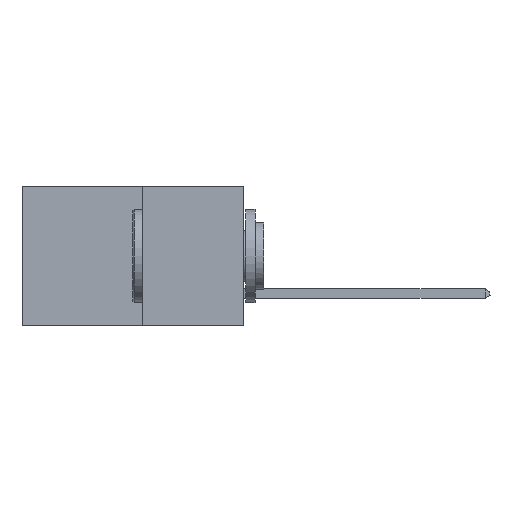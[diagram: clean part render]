
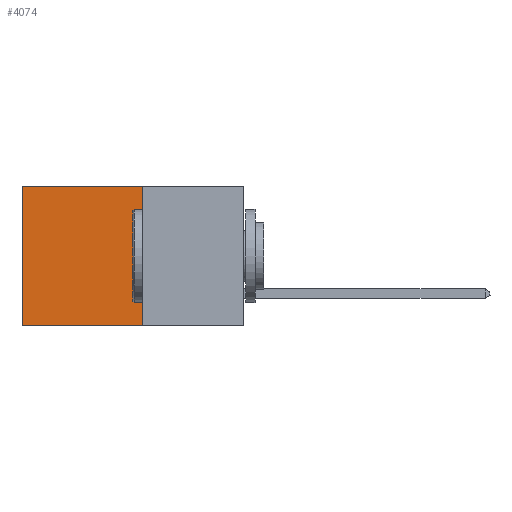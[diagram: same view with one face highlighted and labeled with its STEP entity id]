
A CAD part, left-side view. The second image highlights one B-rep face of the part: STEP entity #4074.
In plain terms, the highlighted planar face has unit normal (-1, 0, 0).
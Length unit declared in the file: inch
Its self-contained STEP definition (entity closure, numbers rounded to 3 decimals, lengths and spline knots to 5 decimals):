
#111 = CARTESIAN_POINT ( 'NONE',  ( 0.277, 0.59, -0.37 ) ) ;
#974 = VERTEX_POINT ( 'NONE', #16463 ) ;
#1836 = ORIENTED_EDGE ( 'NONE', *, *, #10106, .F. ) ;
#2665 = VERTEX_POINT ( 'NONE', #18828 ) ;
#2771 = ORIENTED_EDGE ( 'NONE', *, *, #16842, .F. ) ;
#4074 = ADVANCED_FACE ( 'NONE', ( #10471 ), #6412, .F. ) ;
#4840 = LINE ( 'NONE', #16144, #23337 ) ;
#6259 = DIRECTION ( 'NONE',  ( 0., 0., -1. ) ) ;
#6305 = DIRECTION ( 'NONE',  ( 1., 0., 0. ) ) ;
#6311 = CARTESIAN_POINT ( 'NONE',  ( 0.277, 0.27, -0.37 ) ) ;
#6412 = PLANE ( 'NONE',  #6527 ) ;
#6508 = ORIENTED_EDGE ( 'NONE', *, *, #10746, .T. ) ;
#6527 = AXIS2_PLACEMENT_3D ( 'NONE', #6311, #6305, #6259 ) ;
#7410 = CARTESIAN_POINT ( 'NONE',  ( 0.277, 0.27, -0.37 ) ) ;
#8027 = VECTOR ( 'NONE', #13654, 39.37008 ) ;
#8339 = LINE ( 'NONE', #22713, #22605 ) ;
#8341 = VERTEX_POINT ( 'NONE', #10552 ) ;
#10106 = EDGE_CURVE ( 'NONE', #8341, #14587, #8339, .T. ) ;
#10471 = FACE_OUTER_BOUND ( 'NONE', #18647, .T. ) ;
#10552 = CARTESIAN_POINT ( 'NONE',  ( 0.277, 0.27, 0. ) ) ;
#10746 = EDGE_CURVE ( 'NONE', #8341, #2665, #22304, .T. ) ;
#11811 = ORIENTED_EDGE ( 'NONE', *, *, #18966, .T. ) ;
#13654 = DIRECTION ( 'NONE',  ( 0., 1., 0. ) ) ;
#14587 = VERTEX_POINT ( 'NONE', #7410 ) ;
#14637 = DIRECTION ( 'NONE',  ( 0., 0., -1. ) ) ;
#15468 = CARTESIAN_POINT ( 'NONE',  ( 0.277, 0.27, 0. ) ) ;
#16144 = CARTESIAN_POINT ( 'NONE',  ( 0.277, 0.27, -0.37 ) ) ;
#16463 = CARTESIAN_POINT ( 'NONE',  ( 0.277, 0.59, -0.37 ) ) ;
#16842 = EDGE_CURVE ( 'NONE', #14587, #974, #4840, .T. ) ;
#18009 = LINE ( 'NONE', #111, #21633 ) ;
#18647 = EDGE_LOOP ( 'NONE', ( #11811, #2771, #1836, #6508 ) ) ;
#18828 = CARTESIAN_POINT ( 'NONE',  ( 0.277, 0.59, 0. ) ) ;
#18966 = EDGE_CURVE ( 'NONE', #2665, #974, #18009, .T. ) ;
#19181 = DIRECTION ( 'NONE',  ( 0., 0., -1. ) ) ;
#19182 = DIRECTION ( 'NONE',  ( 0., 1., 0. ) ) ;
#21633 = VECTOR ( 'NONE', #14637, 39.37008 ) ;
#22304 = LINE ( 'NONE', #15468, #8027 ) ;
#22605 = VECTOR ( 'NONE', #19181, 39.37008 ) ;
#22713 = CARTESIAN_POINT ( 'NONE',  ( 0.277, 0.27, -0.37 ) ) ;
#23337 = VECTOR ( 'NONE', #19182, 39.37008 ) ;
